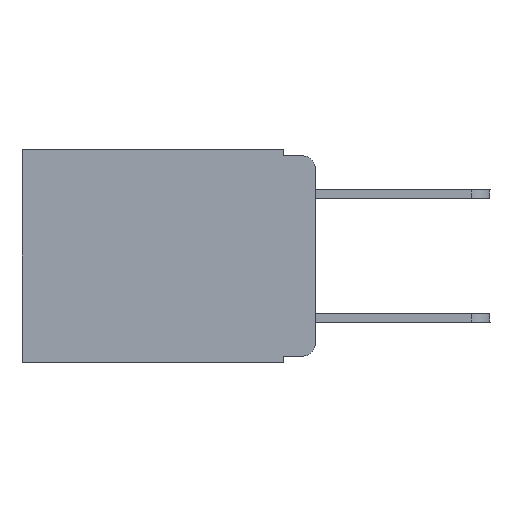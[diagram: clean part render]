
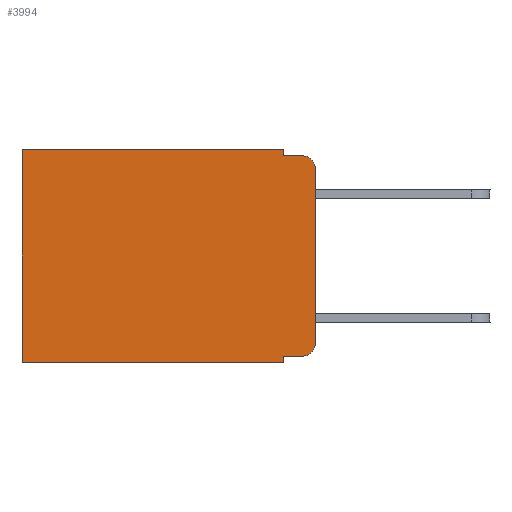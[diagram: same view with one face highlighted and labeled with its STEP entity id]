
A CAD part, left-side view. The second image highlights one B-rep face of the part: STEP entity #3994.
In plain terms, the highlighted planar face has unit normal (-1, 0, 0).
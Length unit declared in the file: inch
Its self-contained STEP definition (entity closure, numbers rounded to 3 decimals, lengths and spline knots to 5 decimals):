
#71 = VERTEX_POINT ( 'NONE', #12096 ) ;
#155 = EDGE_CURVE ( 'NONE', #14241, #13392, #4547, .T. ) ;
#385 = EDGE_CURVE ( 'NONE', #14659, #13392, #2529, .T. ) ;
#559 = CARTESIAN_POINT ( 'NONE',  ( 0.298, 0.473, -0.343 ) ) ;
#651 = ORIENTED_EDGE ( 'NONE', *, *, #14109, .F. ) ;
#724 = ORIENTED_EDGE ( 'NONE', *, *, #5519, .F. ) ;
#753 = LINE ( 'NONE', #14663, #10120 ) ;
#856 = CARTESIAN_POINT ( 'NONE',  ( 0.298, 0.02, -0.03 ) ) ;
#1821 = VERTEX_POINT ( 'NONE', #2075 ) ;
#1913 = CARTESIAN_POINT ( 'NONE',  ( 0.298, 0.051, -0.01 ) ) ;
#2045 = EDGE_CURVE ( 'NONE', #12273, #1821, #14475, .T. ) ;
#2075 = CARTESIAN_POINT ( 'NONE',  ( 0.298, 0.473, 0. ) ) ;
#2529 = LINE ( 'NONE', #6058, #6796 ) ;
#2570 = CARTESIAN_POINT ( 'NONE',  ( 0.298, 0., 0. ) ) ;
#3050 = CARTESIAN_POINT ( 'NONE',  ( 0.298, 0., 0. ) ) ;
#3096 = ORIENTED_EDGE ( 'NONE', *, *, #12707, .T. ) ;
#3234 = ORIENTED_EDGE ( 'NONE', *, *, #155, .T. ) ;
#3274 = EDGE_CURVE ( 'NONE', #71, #5938, #14406, .T. ) ;
#3295 = VERTEX_POINT ( 'NONE', #4969 ) ;
#3476 = EDGE_CURVE ( 'NONE', #8064, #3295, #13906, .T. ) ;
#3619 = ORIENTED_EDGE ( 'NONE', *, *, #3274, .F. ) ;
#3790 = CARTESIAN_POINT ( 'NONE',  ( 0.298, 0.051, 0. ) ) ;
#3994 = ADVANCED_FACE ( 'NONE', ( #12900 ), #14096, .F. ) ;
#4025 = ORIENTED_EDGE ( 'NONE', *, *, #3476, .F. ) ;
#4048 = ORIENTED_EDGE ( 'NONE', *, *, #385, .F. ) ;
#4259 = CARTESIAN_POINT ( 'NONE',  ( 0.298, 0.02, -0.313 ) ) ;
#4295 = ORIENTED_EDGE ( 'NONE', *, *, #5465, .T. ) ;
#4547 = CIRCLE ( 'NONE', #10336, 0.02 ) ;
#4714 = DIRECTION ( 'NONE',  ( 0., 0., -1. ) ) ;
#4961 = CARTESIAN_POINT ( 'NONE',  ( 0.298, 0.051, 0. ) ) ;
#4969 = CARTESIAN_POINT ( 'NONE',  ( 0.298, 0.02, -0.01 ) ) ;
#5287 = DIRECTION ( 'NONE',  ( -1., 0., 0. ) ) ;
#5339 = DIRECTION ( 'NONE',  ( 0., 1., 0. ) ) ;
#5450 = CARTESIAN_POINT ( 'NONE',  ( 0.298, 0.051, 0. ) ) ;
#5465 = EDGE_CURVE ( 'NONE', #14659, #3295, #14233, .T. ) ;
#5519 = EDGE_CURVE ( 'NONE', #5938, #13349, #753, .T. ) ;
#5860 = VECTOR ( 'NONE', #7124, 39.37008 ) ;
#5885 = DIRECTION ( 'NONE',  ( 1., 0., 0. ) ) ;
#5938 = VERTEX_POINT ( 'NONE', #13540 ) ;
#5994 = DIRECTION ( 'NONE',  ( 0., -1., 0. ) ) ;
#6058 = CARTESIAN_POINT ( 'NONE',  ( 0.298, 0., 0. ) ) ;
#6796 = VECTOR ( 'NONE', #4714, 39.37008 ) ;
#6880 = CARTESIAN_POINT ( 'NONE',  ( 0.298, 0.051, -0.01 ) ) ;
#7124 = DIRECTION ( 'NONE',  ( 0., 0., -1. ) ) ;
#7316 = EDGE_CURVE ( 'NONE', #1821, #13349, #7723, .T. ) ;
#7723 = LINE ( 'NONE', #8920, #11008 ) ;
#8064 = VERTEX_POINT ( 'NONE', #1913 ) ;
#8612 = CARTESIAN_POINT ( 'NONE',  ( 0.298, 0., -0.03 ) ) ;
#8633 = DIRECTION ( 'NONE',  ( 0., 0., -1. ) ) ;
#8867 = DIRECTION ( 'NONE',  ( -1., 0., 0. ) ) ;
#8920 = CARTESIAN_POINT ( 'NONE',  ( 0.298, 0.473, 0. ) ) ;
#9192 = AXIS2_PLACEMENT_3D ( 'NONE', #856, #5287, #11104 ) ;
#9391 = LINE ( 'NONE', #10743, #13032 ) ;
#9524 = AXIS2_PLACEMENT_3D ( 'NONE', #2570, #5885, #9583 ) ;
#9583 = DIRECTION ( 'NONE',  ( 0., 0., -1. ) ) ;
#10061 = CARTESIAN_POINT ( 'NONE',  ( 0.298, 0.02, -0.333 ) ) ;
#10120 = VECTOR ( 'NONE', #5339, 39.37008 ) ;
#10336 = AXIS2_PLACEMENT_3D ( 'NONE', #4259, #8867, #10914 ) ;
#10743 = CARTESIAN_POINT ( 'NONE',  ( 0.298, 0.051, -0.333 ) ) ;
#10914 = DIRECTION ( 'NONE',  ( 0., 0., -1. ) ) ;
#10951 = CARTESIAN_POINT ( 'NONE',  ( 0.298, 0., -0.313 ) ) ;
#11008 = VECTOR ( 'NONE', #14781, 39.37008 ) ;
#11104 = DIRECTION ( 'NONE',  ( 0., 0., -1. ) ) ;
#11154 = VECTOR ( 'NONE', #8633, 39.37008 ) ;
#11449 = VECTOR ( 'NONE', #13701, 39.37008 ) ;
#11935 = ORIENTED_EDGE ( 'NONE', *, *, #7316, .T. ) ;
#12096 = CARTESIAN_POINT ( 'NONE',  ( 0.298, 0.051, -0.333 ) ) ;
#12273 = VERTEX_POINT ( 'NONE', #4961 ) ;
#12673 = ORIENTED_EDGE ( 'NONE', *, *, #2045, .T. ) ;
#12707 = EDGE_CURVE ( 'NONE', #71, #14241, #9391, .T. ) ;
#12900 = FACE_OUTER_BOUND ( 'NONE', #14541, .T. ) ;
#13032 = VECTOR ( 'NONE', #5994, 39.37008 ) ;
#13140 = VECTOR ( 'NONE', #14397, 39.37008 ) ;
#13349 = VERTEX_POINT ( 'NONE', #559 ) ;
#13392 = VERTEX_POINT ( 'NONE', #10951 ) ;
#13540 = CARTESIAN_POINT ( 'NONE',  ( 0.298, 0.051, -0.343 ) ) ;
#13701 = DIRECTION ( 'NONE',  ( 0., -1., 0. ) ) ;
#13906 = LINE ( 'NONE', #6880, #11449 ) ;
#14096 = PLANE ( 'NONE',  #9524 ) ;
#14109 = EDGE_CURVE ( 'NONE', #12273, #8064, #14267, .T. ) ;
#14233 = CIRCLE ( 'NONE', #9192, 0.02 ) ;
#14241 = VERTEX_POINT ( 'NONE', #10061 ) ;
#14267 = LINE ( 'NONE', #3790, #5860 ) ;
#14397 = DIRECTION ( 'NONE',  ( 0., 1., 0. ) ) ;
#14406 = LINE ( 'NONE', #5450, #11154 ) ;
#14475 = LINE ( 'NONE', #3050, #13140 ) ;
#14541 = EDGE_LOOP ( 'NONE', ( #4048, #4295, #4025, #651, #12673, #11935, #724, #3619, #3096, #3234 ) ) ;
#14659 = VERTEX_POINT ( 'NONE', #8612 ) ;
#14663 = CARTESIAN_POINT ( 'NONE',  ( 0.298, 0., -0.343 ) ) ;
#14781 = DIRECTION ( 'NONE',  ( 0., 0., -1. ) ) ;
